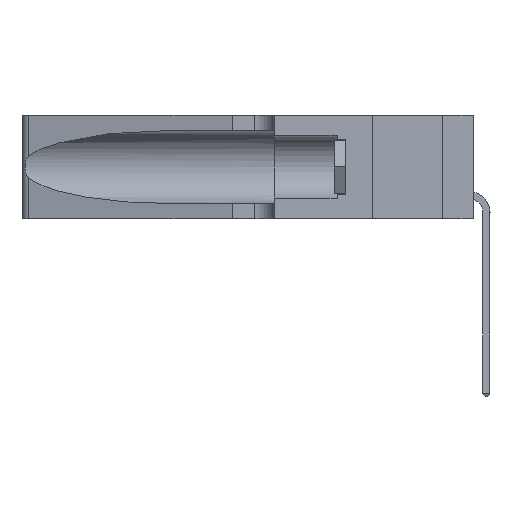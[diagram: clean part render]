
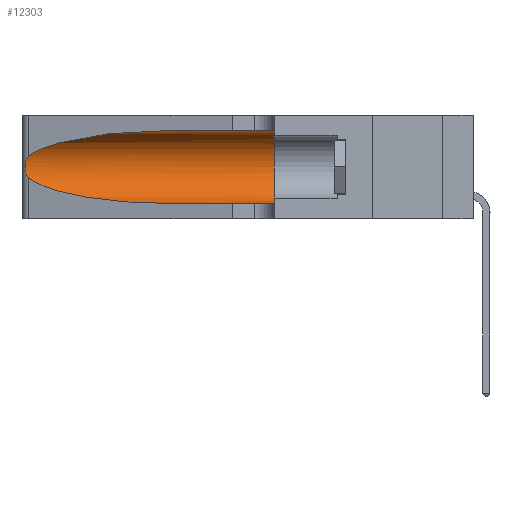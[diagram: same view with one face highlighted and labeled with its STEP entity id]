
A CAD part, left-side view. The second image highlights one B-rep face of the part: STEP entity #12303.
In plain terms, the highlighted cylindrical face has radius 3.308 mm (diameter 6.617 mm), a partial arc.
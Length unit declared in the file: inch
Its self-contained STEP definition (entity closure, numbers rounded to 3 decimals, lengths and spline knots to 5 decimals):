
#701 = FACE_OUTER_BOUND ( 'NONE', #30967, .T. ) ;
#1914 = CARTESIAN_POINT ( 'NONE',  ( 0.18966, 0.96281, 0.05475 ) ) ;
#2586 = EDGE_CURVE ( 'NONE', #30979, #10105, #33555, .T. ) ;
#3651 = CARTESIAN_POINT ( 'NONE',  ( 0.25555, 1.22993, 0.14849 ) ) ;
#5812 = VECTOR ( 'NONE', #28982, 39.37008 ) ;
#6034 = CIRCLE ( 'NONE', #37985, 0.13025 ) ;
#6753 = CYLINDRICAL_SURFACE ( 'NONE', #8235, 0.13025 ) ;
#6918 = B_SPLINE_CURVE_WITH_KNOTS ( 'NONE', 3,
 ( #14334, #7592, #42335, #30367, #11894, #38390, #38551, #27166, #31004, #38073, #8056, #19660, #3651, #15125 ),
 .UNSPECIFIED., .F., .F.,
 ( 4, 2, 2, 2, 2, 2, 4 ),
 ( 0., 0.00027, 0.00053, 0.00107, 0.0016, 0.00187, 0.00214 ),
 .UNSPECIFIED. ) ;
#7592 = CARTESIAN_POINT ( 'NONE',  ( 0.25555, 1.22994, 0.2215 ) ) ;
#7600 = CARTESIAN_POINT ( 'NONE',  ( 0.1305, 1.61858, 0.185 ) ) ;
#8056 = CARTESIAN_POINT ( 'NONE',  ( 0.25789, 1.23486, 0.15765 ) ) ;
#8089 = CARTESIAN_POINT ( 'NONE',  ( 0.1305, 0.35, 0.185 ) ) ;
#8235 = AXIS2_PLACEMENT_3D ( 'NONE', #7600, #31836, #23469 ) ;
#8831 = EDGE_CURVE ( 'NONE', #29362, #12780, #26760, .T. ) ;
#9603 = CARTESIAN_POINT ( 'NONE',  ( 0.1305, 0.72297, 0.31525 ) ) ;
#10105 = VERTEX_POINT ( 'NONE', #32620 ) ;
#11544 = CARTESIAN_POINT ( 'NONE',  ( 0.18966, 0.96281, 0.31525 ) ) ;
#11894 = CARTESIAN_POINT ( 'NONE',  ( 0.25854, 1.2359, 0.20912 ) ) ;
#12303 = ADVANCED_FACE ( 'NONE', ( #701 ), #6753, .F. ) ;
#12780 = VERTEX_POINT ( 'NONE', #29079 ) ;
#14334 = CARTESIAN_POINT ( 'NONE',  ( 0.25487, 1.22718, 0.22369 ) ) ;
#15125 = CARTESIAN_POINT ( 'NONE',  ( 0.25487, 1.22718, 0.14631 ) ) ;
#15747 = ORIENTED_EDGE ( 'NONE', *, *, #40560, .T. ) ;
#17092 = ORIENTED_EDGE ( 'NONE', *, *, #21654, .T. ) ;
#17401 = DIRECTION ( 'NONE',  ( 0., 1., 0. ) ) ;
#18856 = VECTOR ( 'NONE', #37264, 39.37008 ) ;
#19660 = CARTESIAN_POINT ( 'NONE',  ( 0.25639, 1.23186, 0.15144 ) ) ;
#20101 = CARTESIAN_POINT ( 'NONE',  ( 0.1305, 0.35, 0.05475 ) ) ;
#21654 = EDGE_CURVE ( 'NONE', #32950, #30979, #6918, .T. ) ;
#23330 = CARTESIAN_POINT ( 'NONE',  ( 0.25487, 1.22718, 0.22369 ) ) ;
#23469 = DIRECTION ( 'NONE',  ( 0., 0., -1. ) ) ;
#26760 = LINE ( 'NONE', #42449, #5812 ) ;
#26826 = EDGE_CURVE ( 'NONE', #10105, #29453, #46901, .T. ) ;
#27166 = CARTESIAN_POINT ( 'NONE',  ( 0.26075, 1.23896, 0.178 ) ) ;
#28457 = ORIENTED_EDGE ( 'NONE', *, *, #8831, .F. ) ;
#28982 = DIRECTION ( 'NONE',  ( 0., -1., 0. ) ) ;
#29061 = ORIENTED_EDGE ( 'NONE', *, *, #2586, .T. ) ;
#29079 = CARTESIAN_POINT ( 'NONE',  ( 0.1305, 0.35, 0.31525 ) ) ;
#29362 = VERTEX_POINT ( 'NONE', #40878 ) ;
#29453 = VERTEX_POINT ( 'NONE', #20101 ) ;
#30046 = CARTESIAN_POINT ( 'NONE',  ( 0.1305, 1.61858, 0.05475 ) ) ;
#30274 = EDGE_CURVE ( 'NONE', #12780, #29453, #6034, .T. ) ;
#30367 = CARTESIAN_POINT ( 'NONE',  ( 0.25787, 1.23484, 0.2124 ) ) ;
#30967 = EDGE_LOOP ( 'NONE', ( #15747, #17092, #29061, #34085, #31903, #28457 ) ) ;
#30979 = VERTEX_POINT ( 'NONE', #39872 ) ;
#31004 = CARTESIAN_POINT ( 'NONE',  ( 0.26017, 1.23833, 0.17102 ) ) ;
#31120 = CARTESIAN_POINT ( 'NONE',  ( 0.2373, 1.15595, 0.28018 ) ) ;
#31836 = DIRECTION ( 'NONE',  ( 0., -1., 0. ) ) ;
#31903 = ORIENTED_EDGE ( 'NONE', *, *, #30274, .F. ) ;
#32461 = CARTESIAN_POINT ( 'NONE',  ( 0.1305, 0.72297, 0.05475 ) ) ;
#32620 = CARTESIAN_POINT ( 'NONE',  ( 0.1305, 0.72297, 0.05475 ) ) ;
#32950 = VERTEX_POINT ( 'NONE', #23330 ) ;
#33555 =( BOUNDED_CURVE ( )  B_SPLINE_CURVE ( 3, ( #48141, #36142, #1914, #32461 ),
 .UNSPECIFIED., .F., .F. ) 
 B_SPLINE_CURVE_WITH_KNOTS ( ( 4, 4 ),
 ( 3.44316, 4.71239 ),
 .UNSPECIFIED. ) 
 CURVE ( )  GEOMETRIC_REPRESENTATION_ITEM ( )  RATIONAL_B_SPLINE_CURVE ( ( 1., 0.87, 0.87, 1. ) ) 
 REPRESENTATION_ITEM ( '' )  );
#34085 = ORIENTED_EDGE ( 'NONE', *, *, #26826, .T. ) ;
#36142 = CARTESIAN_POINT ( 'NONE',  ( 0.2373, 1.15595, 0.08982 ) ) ;
#37264 = DIRECTION ( 'NONE',  ( 0., -1., 0. ) ) ;
#37985 = AXIS2_PLACEMENT_3D ( 'NONE', #8089, #17401, #39654 ) ;
#38073 = CARTESIAN_POINT ( 'NONE',  ( 0.25856, 1.23593, 0.16098 ) ) ;
#38390 = CARTESIAN_POINT ( 'NONE',  ( 0.26018, 1.23835, 0.19895 ) ) ;
#38551 = CARTESIAN_POINT ( 'NONE',  ( 0.26075, 1.23896, 0.19203 ) ) ;
#39654 = DIRECTION ( 'NONE',  ( 0., 0., 1. ) ) ;
#39872 = CARTESIAN_POINT ( 'NONE',  ( 0.25487, 1.22718, 0.14631 ) ) ;
#40560 = EDGE_CURVE ( 'NONE', #29362, #32950, #44106, .T. ) ;
#40878 = CARTESIAN_POINT ( 'NONE',  ( 0.1305, 0.72297, 0.31525 ) ) ;
#42335 = CARTESIAN_POINT ( 'NONE',  ( 0.25639, 1.23184, 0.21858 ) ) ;
#42449 = CARTESIAN_POINT ( 'NONE',  ( 0.1305, 1.61858, 0.31525 ) ) ;
#44106 =( BOUNDED_CURVE ( )  B_SPLINE_CURVE ( 3, ( #9603, #11544, #31120, #46475 ),
 .UNSPECIFIED., .F., .T. ) 
 B_SPLINE_CURVE_WITH_KNOTS ( ( 4, 4 ),
 ( 1.5708, 2.84003 ),
 .UNSPECIFIED. ) 
 CURVE ( )  GEOMETRIC_REPRESENTATION_ITEM ( )  RATIONAL_B_SPLINE_CURVE ( ( 1., 0.87, 0.87, 1. ) ) 
 REPRESENTATION_ITEM ( '' )  );
#46475 = CARTESIAN_POINT ( 'NONE',  ( 0.25487, 1.22718, 0.22369 ) ) ;
#46901 = LINE ( 'NONE', #30046, #18856 ) ;
#48141 = CARTESIAN_POINT ( 'NONE',  ( 0.25487, 1.22718, 0.14631 ) ) ;
